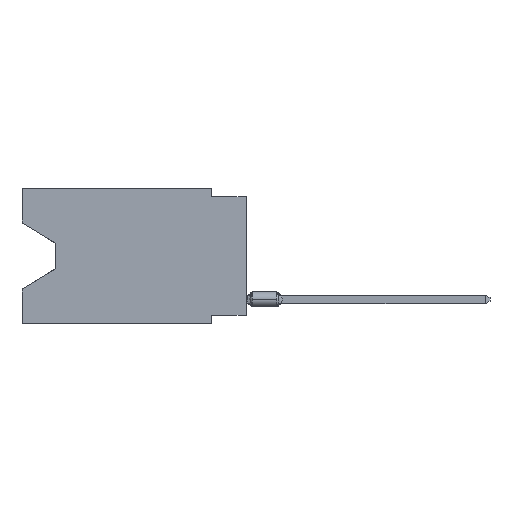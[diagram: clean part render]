
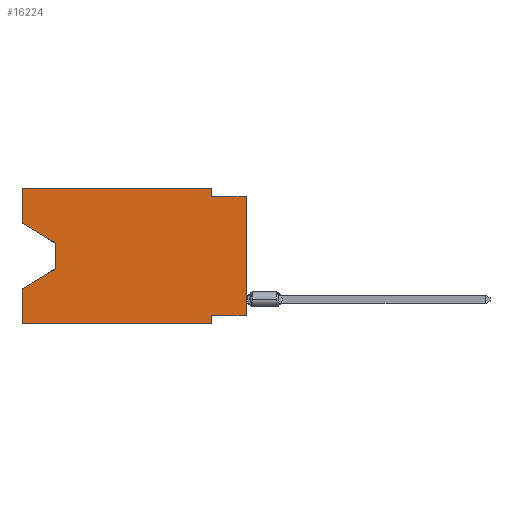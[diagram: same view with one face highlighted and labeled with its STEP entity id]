
A CAD part, left-side view. The second image highlights one B-rep face of the part: STEP entity #16224.
In plain terms, the highlighted planar face has unit normal (-1, 0, 0).
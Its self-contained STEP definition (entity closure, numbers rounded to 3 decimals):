
#101 = ORIENTED_EDGE ( 'NONE', *, *, #9008, .T. ) ;
#251 = DIRECTION ( 'NONE',  ( 0., -1., 0. ) ) ;
#287 = DIRECTION ( 'NONE',  ( 0., -0.855, -0.519 ) ) ;
#1014 = VECTOR ( 'NONE', #5878, 1000. ) ;
#1135 = VERTEX_POINT ( 'NONE', #6462 ) ;
#1149 = ORIENTED_EDGE ( 'NONE', *, *, #9931, .F. ) ;
#1169 = CARTESIAN_POINT ( 'NONE',  ( 0., 16.383, 0. ) ) ;
#1452 = CARTESIAN_POINT ( 'NONE',  ( 0., 13.97, -4.013 ) ) ;
#1462 = EDGE_CURVE ( 'NONE', #19677, #22290, #19921, .T. ) ;
#1744 = DIRECTION ( 'NONE',  ( 1., 0., 0. ) ) ;
#1952 = CARTESIAN_POINT ( 'NONE',  ( 0., 16.383, 0. ) ) ;
#2115 = EDGE_LOOP ( 'NONE', ( #4499, #101, #23045, #21438, #20334, #27269, #1149, #9079, #11220, #10778, #14410, #22320 ) ) ;
#2118 = VECTOR ( 'NONE', #3113, 1000. ) ;
#2187 = EDGE_CURVE ( 'NONE', #3397, #13370, #8019, .T. ) ;
#2366 = LINE ( 'NONE', #19574, #15153 ) ;
#2549 = VERTEX_POINT ( 'NONE', #12624 ) ;
#3113 = DIRECTION ( 'NONE',  ( 0., 1., 0. ) ) ;
#3161 = VECTOR ( 'NONE', #16762, 1000. ) ;
#3397 = VERTEX_POINT ( 'NONE', #20993 ) ;
#3765 = CARTESIAN_POINT ( 'NONE',  ( 0., 2.54, 0. ) ) ;
#3871 = CARTESIAN_POINT ( 'NONE',  ( 0., 16.383, 0. ) ) ;
#4080 = CARTESIAN_POINT ( 'NONE',  ( 0., 16.383, -2.546 ) ) ;
#4232 = DIRECTION ( 'NONE',  ( 0., 0., -1. ) ) ;
#4499 = ORIENTED_EDGE ( 'NONE', *, *, #17148, .T. ) ;
#4554 = DIRECTION ( 'NONE',  ( 0., -1., 0. ) ) ;
#4652 = CARTESIAN_POINT ( 'NONE',  ( 0., 13.97, -4.013 ) ) ;
#5238 = DIRECTION ( 'NONE',  ( 0., 0., -1. ) ) ;
#5633 = LINE ( 'NONE', #12105, #21287 ) ;
#5876 = VECTOR ( 'NONE', #287, 1000. ) ;
#5878 = DIRECTION ( 'NONE',  ( 0., 0., 1. ) ) ;
#6359 = LINE ( 'NONE', #14828, #6474 ) ;
#6435 = EDGE_CURVE ( 'NONE', #2549, #1135, #20692, .T. ) ;
#6462 = CARTESIAN_POINT ( 'NONE',  ( 0., 0., -0.635 ) ) ;
#6474 = VECTOR ( 'NONE', #17751, 1000. ) ;
#7357 = LINE ( 'NONE', #3765, #24970 ) ;
#8016 = CARTESIAN_POINT ( 'NONE',  ( 0., 0., 0. ) ) ;
#8019 = LINE ( 'NONE', #1952, #21852 ) ;
#9008 = EDGE_CURVE ( 'NONE', #12328, #9329, #19119, .T. ) ;
#9064 = CARTESIAN_POINT ( 'NONE',  ( 0., 16.383, -9.906 ) ) ;
#9079 = ORIENTED_EDGE ( 'NONE', *, *, #6435, .T. ) ;
#9228 = VECTOR ( 'NONE', #4554, 1000. ) ;
#9329 = VERTEX_POINT ( 'NONE', #12083 ) ;
#9900 = LINE ( 'NONE', #1169, #13613 ) ;
#9931 = EDGE_CURVE ( 'NONE', #2549, #17155, #17516, .T. ) ;
#10498 = FACE_OUTER_BOUND ( 'NONE', #2115, .T. ) ;
#10778 = ORIENTED_EDGE ( 'NONE', *, *, #22805, .F. ) ;
#10801 = EDGE_CURVE ( 'NONE', #25644, #1135, #2366, .T. ) ;
#10973 = CARTESIAN_POINT ( 'NONE',  ( 0., 2.54, 0. ) ) ;
#11220 = ORIENTED_EDGE ( 'NONE', *, *, #10801, .F. ) ;
#12061 = VECTOR ( 'NONE', #4232, 1000. ) ;
#12083 = CARTESIAN_POINT ( 'NONE',  ( 0., 13.97, -5.893 ) ) ;
#12105 = CARTESIAN_POINT ( 'NONE',  ( 0., 13.97, -5.893 ) ) ;
#12247 = CARTESIAN_POINT ( 'NONE',  ( 0., 2.54, -9.906 ) ) ;
#12328 = VERTEX_POINT ( 'NONE', #1452 ) ;
#12379 = DIRECTION ( 'NONE',  ( 0., 0., 1. ) ) ;
#12391 = LINE ( 'NONE', #12247, #3161 ) ;
#12624 = CARTESIAN_POINT ( 'NONE',  ( 0., 0., -9.271 ) ) ;
#13370 = VERTEX_POINT ( 'NONE', #15458 ) ;
#13591 = CARTESIAN_POINT ( 'NONE',  ( 0., 2.54, -9.906 ) ) ;
#13613 = VECTOR ( 'NONE', #26962, 1000. ) ;
#14410 = ORIENTED_EDGE ( 'NONE', *, *, #19374, .F. ) ;
#14828 = CARTESIAN_POINT ( 'NONE',  ( 0., 16.383, 0. ) ) ;
#15153 = VECTOR ( 'NONE', #251, 1000. ) ;
#15458 = CARTESIAN_POINT ( 'NONE',  ( 0., 16.383, 0. ) ) ;
#15822 = CARTESIAN_POINT ( 'NONE',  ( 0., 16.383, -7.36 ) ) ;
#16224 = ADVANCED_FACE ( 'NONE', ( #10498 ), #16848, .F. ) ;
#16689 = DIRECTION ( 'NONE',  ( 0., 0., -1. ) ) ;
#16762 = DIRECTION ( 'NONE',  ( 0., 0., -1. ) ) ;
#16848 = PLANE ( 'NONE',  #25266 ) ;
#17148 = EDGE_CURVE ( 'NONE', #3397, #12328, #23828, .T. ) ;
#17155 = VERTEX_POINT ( 'NONE', #19742 ) ;
#17516 = LINE ( 'NONE', #26113, #2118 ) ;
#17628 = EDGE_CURVE ( 'NONE', #19677, #27866, #9900, .T. ) ;
#17751 = DIRECTION ( 'NONE',  ( 0., -1., 0. ) ) ;
#17784 = CARTESIAN_POINT ( 'NONE',  ( 0., 2.54, -0.635 ) ) ;
#18738 = VERTEX_POINT ( 'NONE', #10973 ) ;
#19119 = LINE ( 'NONE', #4652, #12061 ) ;
#19374 = EDGE_CURVE ( 'NONE', #13370, #18738, #6359, .T. ) ;
#19574 = CARTESIAN_POINT ( 'NONE',  ( 0., 0., -0.635 ) ) ;
#19677 = VERTEX_POINT ( 'NONE', #20479 ) ;
#19742 = CARTESIAN_POINT ( 'NONE',  ( 0., 2.54, -9.271 ) ) ;
#19921 = LINE ( 'NONE', #9064, #9228 ) ;
#20029 = EDGE_CURVE ( 'NONE', #9329, #27866, #5633, .T. ) ;
#20334 = ORIENTED_EDGE ( 'NONE', *, *, #1462, .T. ) ;
#20479 = CARTESIAN_POINT ( 'NONE',  ( 0., 16.383, -9.906 ) ) ;
#20692 = LINE ( 'NONE', #8016, #1014 ) ;
#20993 = CARTESIAN_POINT ( 'NONE',  ( 0., 16.383, -2.546 ) ) ;
#21287 = VECTOR ( 'NONE', #27037, 1000. ) ;
#21438 = ORIENTED_EDGE ( 'NONE', *, *, #17628, .F. ) ;
#21852 = VECTOR ( 'NONE', #12379, 1000. ) ;
#22290 = VERTEX_POINT ( 'NONE', #13591 ) ;
#22320 = ORIENTED_EDGE ( 'NONE', *, *, #2187, .F. ) ;
#22805 = EDGE_CURVE ( 'NONE', #18738, #25644, #7357, .T. ) ;
#23045 = ORIENTED_EDGE ( 'NONE', *, *, #20029, .T. ) ;
#23828 = LINE ( 'NONE', #4080, #5876 ) ;
#24675 = EDGE_CURVE ( 'NONE', #17155, #22290, #12391, .T. ) ;
#24970 = VECTOR ( 'NONE', #5238, 1000. ) ;
#25266 = AXIS2_PLACEMENT_3D ( 'NONE', #3871, #1744, #16689 ) ;
#25644 = VERTEX_POINT ( 'NONE', #17784 ) ;
#26113 = CARTESIAN_POINT ( 'NONE',  ( 0., 0., -9.271 ) ) ;
#26962 = DIRECTION ( 'NONE',  ( 0., 0., 1. ) ) ;
#27037 = DIRECTION ( 'NONE',  ( 0., 0.855, -0.519 ) ) ;
#27269 = ORIENTED_EDGE ( 'NONE', *, *, #24675, .F. ) ;
#27866 = VERTEX_POINT ( 'NONE', #15822 ) ;
